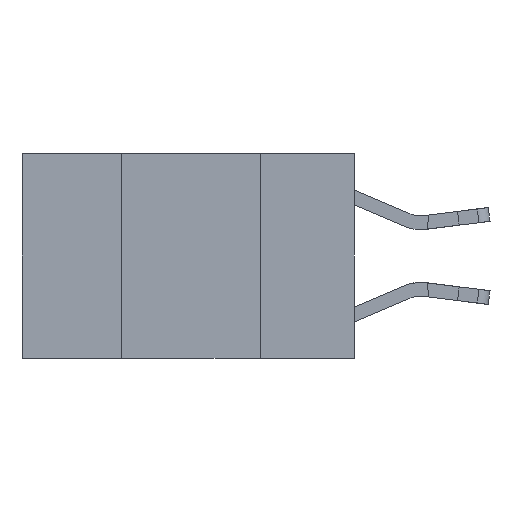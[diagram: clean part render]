
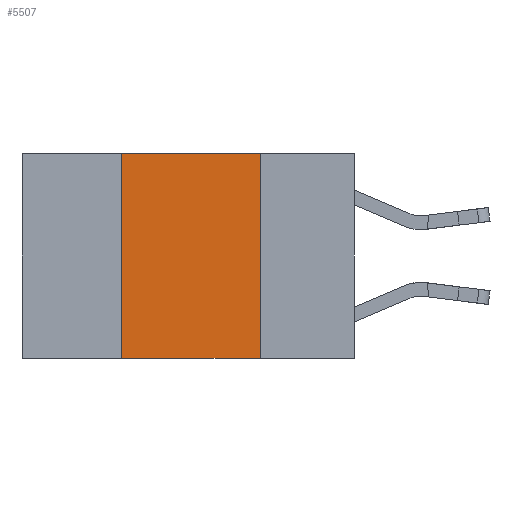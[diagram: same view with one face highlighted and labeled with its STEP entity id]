
A CAD part, left-side view. The second image highlights one B-rep face of the part: STEP entity #5507.
In plain terms, the highlighted planar face has unit normal (-1, 0, 0).
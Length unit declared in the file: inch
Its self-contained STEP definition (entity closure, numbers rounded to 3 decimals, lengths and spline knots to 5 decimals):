
#114 = CARTESIAN_POINT ( 'NONE',  ( 0., 0.42, 0. ) ) ;
#2723 = ORIENTED_EDGE ( 'NONE', *, *, #6802, .F. ) ;
#2857 = LINE ( 'NONE', #17434, #7361 ) ;
#3087 = DIRECTION ( 'NONE',  ( 0., -1., 0. ) ) ;
#4319 = VERTEX_POINT ( 'NONE', #17092 ) ;
#4590 = ORIENTED_EDGE ( 'NONE', *, *, #4903, .F. ) ;
#4863 = DIRECTION ( 'NONE',  ( 0., 0., -1. ) ) ;
#4903 = EDGE_CURVE ( 'NONE', #17949, #17835, #16901, .T. ) ;
#4925 = DIRECTION ( 'NONE',  ( 1., 0., 0. ) ) ;
#5507 = ADVANCED_FACE ( 'NONE', ( #20872 ), #13766, .F. ) ;
#5858 = AXIS2_PLACEMENT_3D ( 'NONE', #15577, #4925, #10272 ) ;
#6037 = ORIENTED_EDGE ( 'NONE', *, *, #18242, .F. ) ;
#6802 = EDGE_CURVE ( 'NONE', #10884, #17949, #13439, .T. ) ;
#7361 = VECTOR ( 'NONE', #3087, 39.37008 ) ;
#9728 = DIRECTION ( 'NONE',  ( 0., 0., 1. ) ) ;
#10272 = DIRECTION ( 'NONE',  ( 0., 0., -1. ) ) ;
#10884 = VERTEX_POINT ( 'NONE', #22402 ) ;
#10921 = CARTESIAN_POINT ( 'NONE',  ( 0., 0.6, 0. ) ) ;
#11976 = ORIENTED_EDGE ( 'NONE', *, *, #12908, .T. ) ;
#12141 = LINE ( 'NONE', #19581, #14363 ) ;
#12908 = EDGE_CURVE ( 'NONE', #10884, #4319, #2857, .T. ) ;
#13439 = LINE ( 'NONE', #22587, #14618 ) ;
#13766 = PLANE ( 'NONE',  #5858 ) ;
#14363 = VECTOR ( 'NONE', #4863, 39.37008 ) ;
#14618 = VECTOR ( 'NONE', #9728, 39.37008 ) ;
#15577 = CARTESIAN_POINT ( 'NONE',  ( 0., 0.6, 0. ) ) ;
#16901 = LINE ( 'NONE', #10921, #21670 ) ;
#17092 = CARTESIAN_POINT ( 'NONE',  ( 0., 0.17, -0.37 ) ) ;
#17434 = CARTESIAN_POINT ( 'NONE',  ( 0., 0.6, -0.37 ) ) ;
#17835 = VERTEX_POINT ( 'NONE', #22145 ) ;
#17949 = VERTEX_POINT ( 'NONE', #114 ) ;
#18232 = DIRECTION ( 'NONE',  ( 0., -1., 0. ) ) ;
#18242 = EDGE_CURVE ( 'NONE', #17835, #4319, #12141, .T. ) ;
#18905 = EDGE_LOOP ( 'NONE', ( #6037, #4590, #2723, #11976 ) ) ;
#19581 = CARTESIAN_POINT ( 'NONE',  ( 0., 0.17, 0. ) ) ;
#20872 = FACE_OUTER_BOUND ( 'NONE', #18905, .T. ) ;
#21670 = VECTOR ( 'NONE', #18232, 39.37008 ) ;
#22145 = CARTESIAN_POINT ( 'NONE',  ( 0., 0.17, 0. ) ) ;
#22402 = CARTESIAN_POINT ( 'NONE',  ( 0., 0.42, -0.37 ) ) ;
#22587 = CARTESIAN_POINT ( 'NONE',  ( 0., 0.42, 0. ) ) ;
